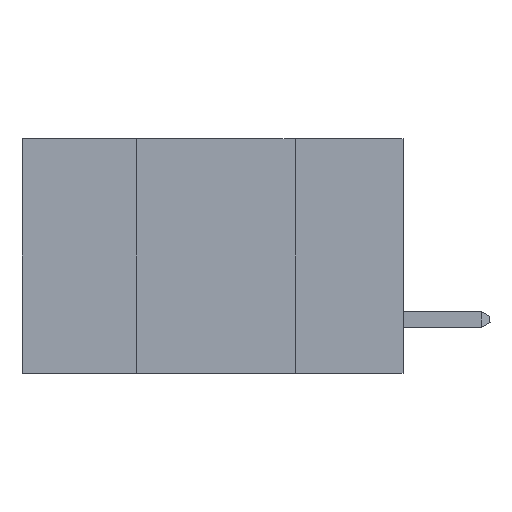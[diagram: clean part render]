
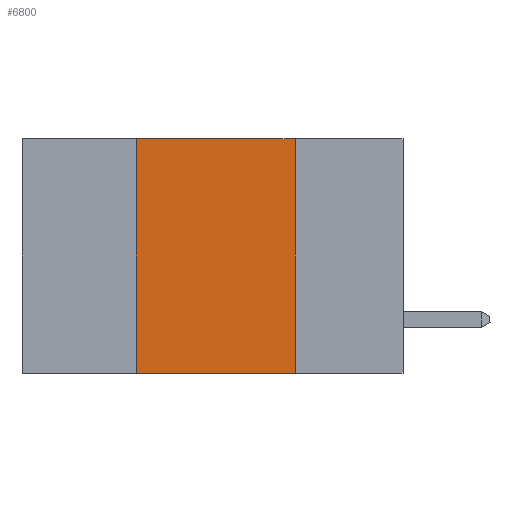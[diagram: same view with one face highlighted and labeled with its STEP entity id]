
A CAD part, left-side view. The second image highlights one B-rep face of the part: STEP entity #6800.
In plain terms, the highlighted planar face has unit normal (-1, 0, 0).
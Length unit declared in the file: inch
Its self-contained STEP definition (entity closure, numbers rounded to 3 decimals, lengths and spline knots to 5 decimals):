
#620 = EDGE_CURVE ( 'NONE', #6413, #2414, #15068, .T. ) ;
#1437 = DIRECTION ( 'NONE',  ( 0., -1., 0. ) ) ;
#2007 = CARTESIAN_POINT ( 'NONE',  ( 0., 0.42, 0. ) ) ;
#2414 = VERTEX_POINT ( 'NONE', #10428 ) ;
#3220 = VERTEX_POINT ( 'NONE', #12934 ) ;
#3367 = DIRECTION ( 'NONE',  ( 0., 0., 1. ) ) ;
#3920 = CARTESIAN_POINT ( 'NONE',  ( 0., 0.42, -0.37 ) ) ;
#4232 = LINE ( 'NONE', #21763, #8344 ) ;
#5089 = DIRECTION ( 'NONE',  ( 0., -1., 0. ) ) ;
#5423 = EDGE_LOOP ( 'NONE', ( #15133, #16642, #7496, #22686 ) ) ;
#6318 = DIRECTION ( 'NONE',  ( 1., 0., 0. ) ) ;
#6413 = VERTEX_POINT ( 'NONE', #2007 ) ;
#6451 = FACE_OUTER_BOUND ( 'NONE', #5423, .T. ) ;
#6800 = ADVANCED_FACE ( 'NONE', ( #6451 ), #16414, .F. ) ;
#7496 = ORIENTED_EDGE ( 'NONE', *, *, #11798, .F. ) ;
#8344 = VECTOR ( 'NONE', #25558, 39.37008 ) ;
#8865 = EDGE_CURVE ( 'NONE', #14074, #3220, #24083, .T. ) ;
#9501 = VECTOR ( 'NONE', #1437, 39.37008 ) ;
#10428 = CARTESIAN_POINT ( 'NONE',  ( 0., 0.17, 0. ) ) ;
#11798 = EDGE_CURVE ( 'NONE', #14074, #6413, #17314, .T. ) ;
#12177 = VECTOR ( 'NONE', #3367, 39.37008 ) ;
#12934 = CARTESIAN_POINT ( 'NONE',  ( 0., 0.17, -0.37 ) ) ;
#14074 = VERTEX_POINT ( 'NONE', #3920 ) ;
#15068 = LINE ( 'NONE', #25574, #21439 ) ;
#15133 = ORIENTED_EDGE ( 'NONE', *, *, #23032, .F. ) ;
#16327 = CARTESIAN_POINT ( 'NONE',  ( 0., 0.6, 0. ) ) ;
#16414 = PLANE ( 'NONE',  #22064 ) ;
#16642 = ORIENTED_EDGE ( 'NONE', *, *, #620, .F. ) ;
#17314 = LINE ( 'NONE', #23711, #12177 ) ;
#19431 = CARTESIAN_POINT ( 'NONE',  ( 0., 0.6, -0.37 ) ) ;
#21439 = VECTOR ( 'NONE', #5089, 39.37008 ) ;
#21763 = CARTESIAN_POINT ( 'NONE',  ( 0., 0.17, 0. ) ) ;
#22064 = AXIS2_PLACEMENT_3D ( 'NONE', #16327, #6318, #24282 ) ;
#22686 = ORIENTED_EDGE ( 'NONE', *, *, #8865, .T. ) ;
#23032 = EDGE_CURVE ( 'NONE', #2414, #3220, #4232, .T. ) ;
#23711 = CARTESIAN_POINT ( 'NONE',  ( 0., 0.42, 0. ) ) ;
#24083 = LINE ( 'NONE', #19431, #9501 ) ;
#24282 = DIRECTION ( 'NONE',  ( 0., 0., -1. ) ) ;
#25558 = DIRECTION ( 'NONE',  ( 0., 0., -1. ) ) ;
#25574 = CARTESIAN_POINT ( 'NONE',  ( 0., 0.6, 0. ) ) ;
